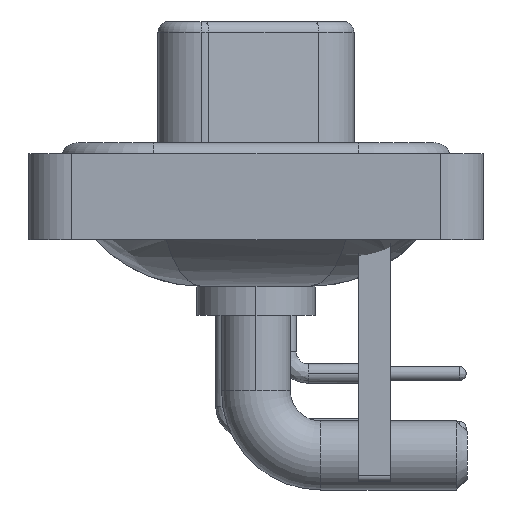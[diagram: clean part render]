
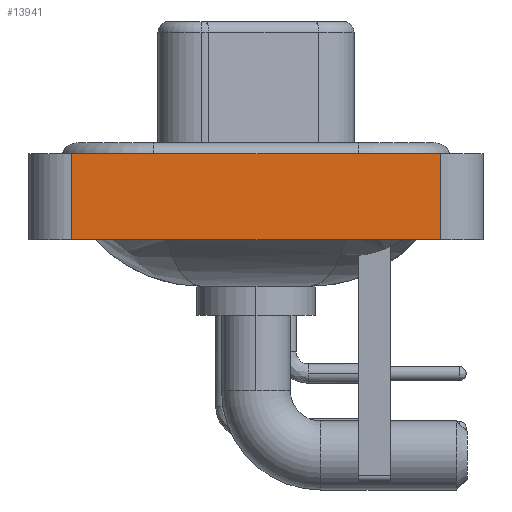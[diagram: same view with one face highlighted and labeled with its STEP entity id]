
A CAD part, left-side view. The second image highlights one B-rep face of the part: STEP entity #13941.
In plain terms, the highlighted planar face has unit normal (-1, 0, 0).
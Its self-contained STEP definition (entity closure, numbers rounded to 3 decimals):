
#583 = LINE ( 'NONE', #13750, #21089 ) ;
#852 = EDGE_CURVE ( 'NONE', #9825, #7084, #17773, .T. ) ;
#1332 = LINE ( 'NONE', #6048, #27229 ) ;
#2756 = PLANE ( 'NONE',  #14205 ) ;
#3186 = DIRECTION ( 'NONE',  ( -1., 0., 0. ) ) ;
#6048 = CARTESIAN_POINT ( 'NONE',  ( -7.35, -8.55, -3.6 ) ) ;
#7084 = VERTEX_POINT ( 'NONE', #16328 ) ;
#7514 = EDGE_LOOP ( 'NONE', ( #22031, #26496, #16402, #21227 ) ) ;
#7551 = VERTEX_POINT ( 'NONE', #8565 ) ;
#7930 = VECTOR ( 'NONE', #20577, 1000. ) ;
#8565 = CARTESIAN_POINT ( 'NONE',  ( -7.35, -8.55, 0.4 ) ) ;
#9825 = VERTEX_POINT ( 'NONE', #26267 ) ;
#11135 = CARTESIAN_POINT ( 'NONE',  ( -7.35, -8.55, -3.6 ) ) ;
#11871 = EDGE_CURVE ( 'NONE', #9825, #14149, #1332, .T. ) ;
#12397 = CARTESIAN_POINT ( 'NONE',  ( -7.35, -8.55, -3.6 ) ) ;
#13750 = CARTESIAN_POINT ( 'NONE',  ( -7.35, -8.55, 0.4 ) ) ;
#13941 = ADVANCED_FACE ( 'NONE', ( #25783 ), #2756, .T. ) ;
#14149 = VERTEX_POINT ( 'NONE', #11135 ) ;
#14205 = AXIS2_PLACEMENT_3D ( 'NONE', #12397, #3186, #14315 ) ;
#14315 = DIRECTION ( 'NONE',  ( 0., 0., 1. ) ) ;
#16328 = CARTESIAN_POINT ( 'NONE',  ( -7.35, 8.55, 0.4 ) ) ;
#16402 = ORIENTED_EDGE ( 'NONE', *, *, #852, .F. ) ;
#17773 = LINE ( 'NONE', #23824, #27300 ) ;
#20577 = DIRECTION ( 'NONE',  ( 0., 0., 1. ) ) ;
#21089 = VECTOR ( 'NONE', #23313, 1000. ) ;
#21227 = ORIENTED_EDGE ( 'NONE', *, *, #11871, .T. ) ;
#21859 = EDGE_CURVE ( 'NONE', #7084, #7551, #583, .T. ) ;
#21905 = DIRECTION ( 'NONE',  ( 0., 0., 1. ) ) ;
#22031 = ORIENTED_EDGE ( 'NONE', *, *, #29100, .T. ) ;
#22632 = CARTESIAN_POINT ( 'NONE',  ( -7.35, -8.55, -3.6 ) ) ;
#22776 = LINE ( 'NONE', #22632, #7930 ) ;
#23313 = DIRECTION ( 'NONE',  ( 0., -1., 0. ) ) ;
#23824 = CARTESIAN_POINT ( 'NONE',  ( -7.35, 8.55, -3.6 ) ) ;
#25783 = FACE_OUTER_BOUND ( 'NONE', #7514, .T. ) ;
#26132 = DIRECTION ( 'NONE',  ( 0., -1., 0. ) ) ;
#26267 = CARTESIAN_POINT ( 'NONE',  ( -7.35, 8.55, -3.6 ) ) ;
#26496 = ORIENTED_EDGE ( 'NONE', *, *, #21859, .F. ) ;
#27229 = VECTOR ( 'NONE', #26132, 1000. ) ;
#27300 = VECTOR ( 'NONE', #21905, 1000. ) ;
#29100 = EDGE_CURVE ( 'NONE', #14149, #7551, #22776, .T. ) ;
